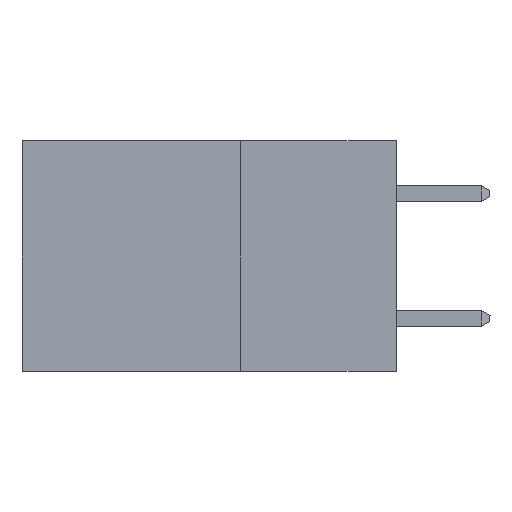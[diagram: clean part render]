
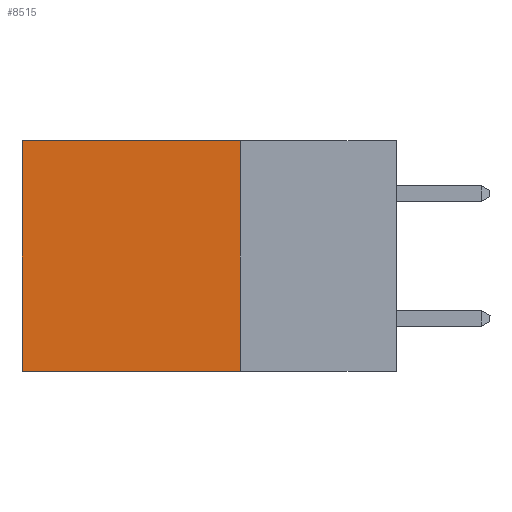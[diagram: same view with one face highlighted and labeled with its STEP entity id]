
A CAD part, left-side view. The second image highlights one B-rep face of the part: STEP entity #8515.
In plain terms, the highlighted planar face has unit normal (-1, 0, 0).
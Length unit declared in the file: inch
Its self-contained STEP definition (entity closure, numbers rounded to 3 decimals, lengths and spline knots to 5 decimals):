
#53 = EDGE_CURVE ( 'NONE', #3754, #20154, #20725, .T. ) ;
#85 = CARTESIAN_POINT ( 'NONE',  ( 0.2615, 0.25, -0.37 ) ) ;
#514 = CARTESIAN_POINT ( 'NONE',  ( 0.2615, 0.25, 0. ) ) ;
#1235 = CARTESIAN_POINT ( 'NONE',  ( 0.2615, 0.25, -0.37 ) ) ;
#1287 = VERTEX_POINT ( 'NONE', #15367 ) ;
#3074 = DIRECTION ( 'NONE',  ( 0., 1., 0. ) ) ;
#3383 = EDGE_CURVE ( 'NONE', #20154, #1287, #10426, .T. ) ;
#3651 = FACE_OUTER_BOUND ( 'NONE', #17262, .T. ) ;
#3754 = VERTEX_POINT ( 'NONE', #514 ) ;
#4503 = ORIENTED_EDGE ( 'NONE', *, *, #9839, .T. ) ;
#4505 = DIRECTION ( 'NONE',  ( 0., 0., -1. ) ) ;
#4645 = LINE ( 'NONE', #8697, #8970 ) ;
#5409 = DIRECTION ( 'NONE',  ( 0., 0., -1. ) ) ;
#5801 = VECTOR ( 'NONE', #3074, 39.37008 ) ;
#7265 = CARTESIAN_POINT ( 'NONE',  ( 0.2615, 0.6, 0. ) ) ;
#8515 = ADVANCED_FACE ( 'NONE', ( #3651 ), #12591, .F. ) ;
#8697 = CARTESIAN_POINT ( 'NONE',  ( 0.2615, 0.6, -0.37 ) ) ;
#8883 = EDGE_CURVE ( 'NONE', #12481, #1287, #4645, .T. ) ;
#8970 = VECTOR ( 'NONE', #5409, 39.37008 ) ;
#9839 = EDGE_CURVE ( 'NONE', #3754, #12481, #13919, .T. ) ;
#10426 = LINE ( 'NONE', #85, #15259 ) ;
#11261 = AXIS2_PLACEMENT_3D ( 'NONE', #1235, #14224, #4505 ) ;
#11734 = CARTESIAN_POINT ( 'NONE',  ( 0.2615, 0.25, -0.37 ) ) ;
#11751 = ORIENTED_EDGE ( 'NONE', *, *, #3383, .F. ) ;
#12481 = VERTEX_POINT ( 'NONE', #7265 ) ;
#12591 = PLANE ( 'NONE',  #11261 ) ;
#13047 = ORIENTED_EDGE ( 'NONE', *, *, #8883, .T. ) ;
#13919 = LINE ( 'NONE', #17580, #5801 ) ;
#14224 = DIRECTION ( 'NONE',  ( 1., 0., 0. ) ) ;
#15259 = VECTOR ( 'NONE', #20500, 39.37008 ) ;
#15367 = CARTESIAN_POINT ( 'NONE',  ( 0.2615, 0.6, -0.37 ) ) ;
#16526 = VECTOR ( 'NONE', #18674, 39.37008 ) ;
#17137 = CARTESIAN_POINT ( 'NONE',  ( 0.2615, 0.25, -0.37 ) ) ;
#17262 = EDGE_LOOP ( 'NONE', ( #13047, #11751, #19836, #4503 ) ) ;
#17580 = CARTESIAN_POINT ( 'NONE',  ( 0.2615, 0.25, 0. ) ) ;
#18674 = DIRECTION ( 'NONE',  ( 0., 0., -1. ) ) ;
#19836 = ORIENTED_EDGE ( 'NONE', *, *, #53, .F. ) ;
#20154 = VERTEX_POINT ( 'NONE', #11734 ) ;
#20500 = DIRECTION ( 'NONE',  ( 0., 1., 0. ) ) ;
#20725 = LINE ( 'NONE', #17137, #16526 ) ;
